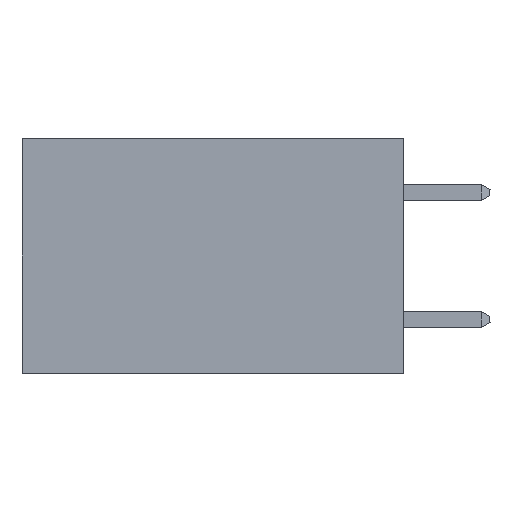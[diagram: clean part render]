
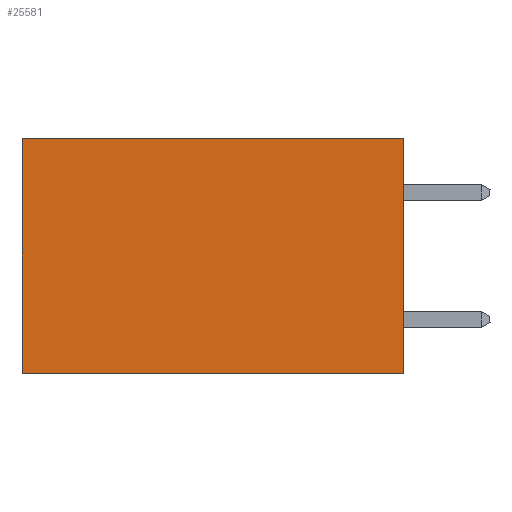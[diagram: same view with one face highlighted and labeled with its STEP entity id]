
A CAD part, left-side view. The second image highlights one B-rep face of the part: STEP entity #25581.
In plain terms, the highlighted planar face has unit normal (-1, 0, 0).
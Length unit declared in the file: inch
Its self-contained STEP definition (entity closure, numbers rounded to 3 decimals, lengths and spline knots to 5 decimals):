
#2613 = DIRECTION ( 'NONE',  ( 0., 0., -1. ) ) ;
#2785 = EDGE_CURVE ( 'NONE', #35007, #29727, #28992, .T. ) ;
#3970 = DIRECTION ( 'NONE',  ( 0., 0., -1. ) ) ;
#5308 = EDGE_CURVE ( 'NONE', #21081, #29727, #37601, .T. ) ;
#7360 = EDGE_LOOP ( 'NONE', ( #38131, #33769, #21330, #16194 ) ) ;
#8453 = CARTESIAN_POINT ( 'NONE',  ( 0.2875, 0.6, 0. ) ) ;
#9446 = AXIS2_PLACEMENT_3D ( 'NONE', #44278, #23641, #2613 ) ;
#10360 = VECTOR ( 'NONE', #12019, 39.37008 ) ;
#12019 = DIRECTION ( 'NONE',  ( 0., 1., 0. ) ) ;
#13870 = CARTESIAN_POINT ( 'NONE',  ( 0.2875, 0., 0. ) ) ;
#14229 = VERTEX_POINT ( 'NONE', #27083 ) ;
#15295 = LINE ( 'NONE', #13870, #32778 ) ;
#16194 = ORIENTED_EDGE ( 'NONE', *, *, #31050, .T. ) ;
#16373 = EDGE_CURVE ( 'NONE', #14229, #35007, #39326, .T. ) ;
#17553 = VECTOR ( 'NONE', #3970, 39.37008 ) ;
#20263 = VECTOR ( 'NONE', #36327, 39.37008 ) ;
#21081 = VERTEX_POINT ( 'NONE', #35714 ) ;
#21218 = CARTESIAN_POINT ( 'NONE',  ( 0.2875, 0., -0.37 ) ) ;
#21330 = ORIENTED_EDGE ( 'NONE', *, *, #16373, .F. ) ;
#23641 = DIRECTION ( 'NONE',  ( 1., 0., 0. ) ) ;
#25581 = ADVANCED_FACE ( 'NONE', ( #42671 ), #30437, .F. ) ;
#27083 = CARTESIAN_POINT ( 'NONE',  ( 0.2875, 0., 0. ) ) ;
#28433 = CARTESIAN_POINT ( 'NONE',  ( 0.2875, 0., 0. ) ) ;
#28992 = LINE ( 'NONE', #42980, #10360 ) ;
#29727 = VERTEX_POINT ( 'NONE', #41280 ) ;
#30437 = PLANE ( 'NONE',  #9446 ) ;
#31050 = EDGE_CURVE ( 'NONE', #14229, #21081, #15295, .T. ) ;
#32778 = VECTOR ( 'NONE', #38203, 39.37008 ) ;
#33769 = ORIENTED_EDGE ( 'NONE', *, *, #2785, .F. ) ;
#35007 = VERTEX_POINT ( 'NONE', #21218 ) ;
#35714 = CARTESIAN_POINT ( 'NONE',  ( 0.2875, 0.6, 0. ) ) ;
#36327 = DIRECTION ( 'NONE',  ( 0., 0., -1. ) ) ;
#37601 = LINE ( 'NONE', #8453, #20263 ) ;
#38131 = ORIENTED_EDGE ( 'NONE', *, *, #5308, .T. ) ;
#38203 = DIRECTION ( 'NONE',  ( 0., 1., 0. ) ) ;
#39326 = LINE ( 'NONE', #28433, #17553 ) ;
#41280 = CARTESIAN_POINT ( 'NONE',  ( 0.2875, 0.6, -0.37 ) ) ;
#42671 = FACE_OUTER_BOUND ( 'NONE', #7360, .T. ) ;
#42980 = CARTESIAN_POINT ( 'NONE',  ( 0.2875, 0., -0.37 ) ) ;
#44278 = CARTESIAN_POINT ( 'NONE',  ( 0.2875, 0., 0. ) ) ;
